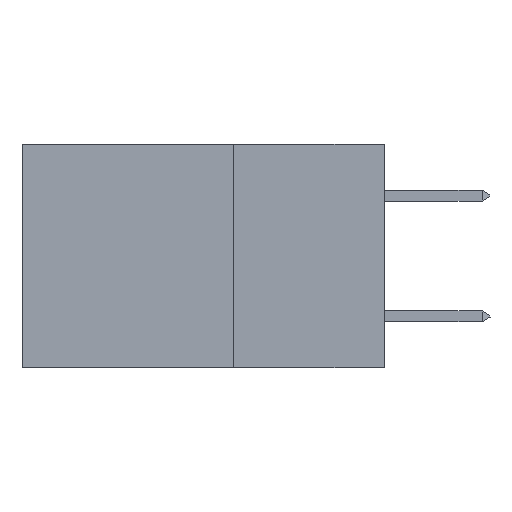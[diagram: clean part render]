
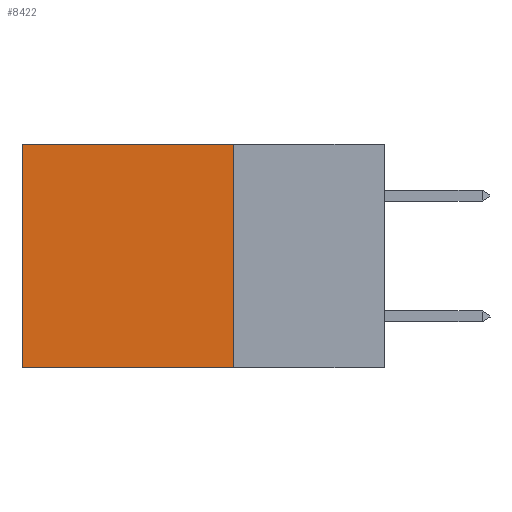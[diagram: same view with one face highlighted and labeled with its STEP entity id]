
A CAD part, left-side view. The second image highlights one B-rep face of the part: STEP entity #8422.
In plain terms, the highlighted planar face has unit normal (-1, 0, 0).
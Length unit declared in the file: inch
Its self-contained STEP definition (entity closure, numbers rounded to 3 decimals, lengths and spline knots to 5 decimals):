
#473 = VERTEX_POINT ( 'NONE', #13012 ) ;
#493 = VERTEX_POINT ( 'NONE', #15550 ) ;
#1016 = LINE ( 'NONE', #16109, #14538 ) ;
#1111 = DIRECTION ( 'NONE',  ( 0., 0., -1. ) ) ;
#1755 = ORIENTED_EDGE ( 'NONE', *, *, #6186, .T. ) ;
#2247 = AXIS2_PLACEMENT_3D ( 'NONE', #15406, #3204, #9661 ) ;
#2555 = VECTOR ( 'NONE', #1111, 39.37008 ) ;
#2853 = DIRECTION ( 'NONE',  ( 0., 0., -1. ) ) ;
#3204 = DIRECTION ( 'NONE',  ( 1., 0., 0. ) ) ;
#3464 = VECTOR ( 'NONE', #9388, 39.37008 ) ;
#3530 = CARTESIAN_POINT ( 'NONE',  ( 0.2875, 0.25, 0. ) ) ;
#3842 = LINE ( 'NONE', #6207, #3464 ) ;
#4358 = CARTESIAN_POINT ( 'NONE',  ( 0.2875, 0.25, 0. ) ) ;
#4769 = EDGE_CURVE ( 'NONE', #7274, #473, #12980, .T. ) ;
#5927 = EDGE_LOOP ( 'NONE', ( #1755, #6592, #15588, #6075 ) ) ;
#6075 = ORIENTED_EDGE ( 'NONE', *, *, #4769, .T. ) ;
#6186 = EDGE_CURVE ( 'NONE', #473, #8251, #11188, .T. ) ;
#6207 = CARTESIAN_POINT ( 'NONE',  ( 0.2875, 0.25, -0.37 ) ) ;
#6250 = EDGE_CURVE ( 'NONE', #7274, #493, #1016, .T. ) ;
#6592 = ORIENTED_EDGE ( 'NONE', *, *, #7440, .F. ) ;
#7274 = VERTEX_POINT ( 'NONE', #3530 ) ;
#7284 = CARTESIAN_POINT ( 'NONE',  ( 0.2875, 0.6, 0. ) ) ;
#7440 = EDGE_CURVE ( 'NONE', #493, #8251, #3842, .T. ) ;
#8251 = VERTEX_POINT ( 'NONE', #8733 ) ;
#8422 = ADVANCED_FACE ( 'NONE', ( #8774 ), #13140, .F. ) ;
#8733 = CARTESIAN_POINT ( 'NONE',  ( 0.2875, 0.6, -0.37 ) ) ;
#8774 = FACE_OUTER_BOUND ( 'NONE', #5927, .T. ) ;
#9388 = DIRECTION ( 'NONE',  ( 0., 1., 0. ) ) ;
#9661 = DIRECTION ( 'NONE',  ( 0., 0., -1. ) ) ;
#11188 = LINE ( 'NONE', #7284, #2555 ) ;
#12220 = VECTOR ( 'NONE', #13149, 39.37008 ) ;
#12980 = LINE ( 'NONE', #4358, #12220 ) ;
#13012 = CARTESIAN_POINT ( 'NONE',  ( 0.2875, 0.6, 0. ) ) ;
#13140 = PLANE ( 'NONE',  #2247 ) ;
#13149 = DIRECTION ( 'NONE',  ( 0., 1., 0. ) ) ;
#14538 = VECTOR ( 'NONE', #2853, 39.37008 ) ;
#15406 = CARTESIAN_POINT ( 'NONE',  ( 0.2875, 0.25, 0. ) ) ;
#15550 = CARTESIAN_POINT ( 'NONE',  ( 0.2875, 0.25, -0.37 ) ) ;
#15588 = ORIENTED_EDGE ( 'NONE', *, *, #6250, .F. ) ;
#16109 = CARTESIAN_POINT ( 'NONE',  ( 0.2875, 0.25, 0. ) ) ;
